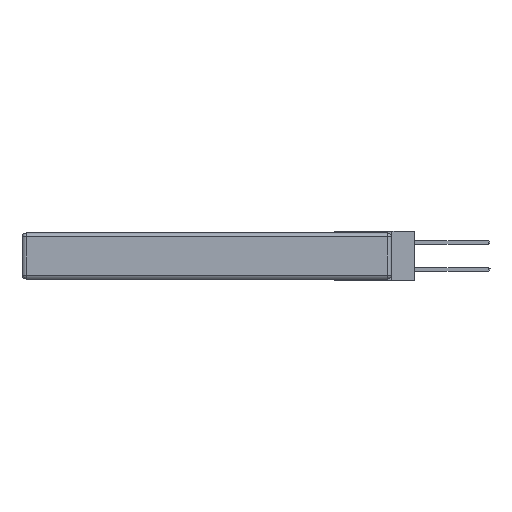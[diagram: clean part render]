
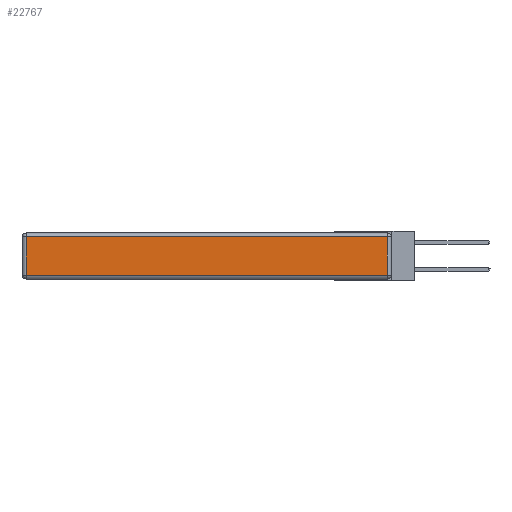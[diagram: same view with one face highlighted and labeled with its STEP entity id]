
A CAD part, left-side view. The second image highlights one B-rep face of the part: STEP entity #22767.
In plain terms, the highlighted planar face has unit normal (-1, 0, 0).
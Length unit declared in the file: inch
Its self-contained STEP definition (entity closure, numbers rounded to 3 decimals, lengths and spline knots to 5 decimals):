
#1443 = VERTEX_POINT ( 'NONE', #26901 ) ;
#3291 = VERTEX_POINT ( 'NONE', #21496 ) ;
#3654 = VECTOR ( 'NONE', #13012, 39.37008 ) ;
#5261 = VERTEX_POINT ( 'NONE', #15467 ) ;
#6190 = EDGE_CURVE ( 'NONE', #3291, #5261, #28071, .T. ) ;
#6710 = PLANE ( 'NONE',  #21973 ) ;
#7044 = CARTESIAN_POINT ( 'NONE',  ( 0., 0., -0.313 ) ) ;
#7120 = DIRECTION ( 'NONE',  ( -1., 0., 0. ) ) ;
#8786 = ORIENTED_EDGE ( 'NONE', *, *, #29482, .T. ) ;
#8874 = EDGE_LOOP ( 'NONE', ( #8786, #17378, #11935, #13070 ) ) ;
#9008 = EDGE_CURVE ( 'NONE', #1443, #3291, #22227, .T. ) ;
#9348 = CARTESIAN_POINT ( 'NONE',  ( 0., 0., -0.343 ) ) ;
#9771 = DIRECTION ( 'NONE',  ( 0., -1., 0. ) ) ;
#11935 = ORIENTED_EDGE ( 'NONE', *, *, #9008, .T. ) ;
#11983 = LINE ( 'NONE', #7044, #22804 ) ;
#13012 = DIRECTION ( 'NONE',  ( 0., 0., 1. ) ) ;
#13070 = ORIENTED_EDGE ( 'NONE', *, *, #6190, .T. ) ;
#13117 = DIRECTION ( 'NONE',  ( 0., 1., 0. ) ) ;
#13322 = CARTESIAN_POINT ( 'NONE',  ( 0., 2.75, -0.03 ) ) ;
#15467 = CARTESIAN_POINT ( 'NONE',  ( 0., 2.72, -0.313 ) ) ;
#17378 = ORIENTED_EDGE ( 'NONE', *, *, #17575, .T. ) ;
#17575 = EDGE_CURVE ( 'NONE', #27498, #1443, #22756, .T. ) ;
#19039 = DIRECTION ( 'NONE',  ( 0., 0., -1. ) ) ;
#21023 = CARTESIAN_POINT ( 'NONE',  ( 0., 2.72, -0.343 ) ) ;
#21474 = VECTOR ( 'NONE', #13117, 39.37008 ) ;
#21496 = CARTESIAN_POINT ( 'NONE',  ( 0., 2.72, -0.03 ) ) ;
#21973 = AXIS2_PLACEMENT_3D ( 'NONE', #9348, #7120, #25855 ) ;
#22227 = LINE ( 'NONE', #13322, #21474 ) ;
#22756 = LINE ( 'NONE', #27522, #3654 ) ;
#22767 = ADVANCED_FACE ( 'NONE', ( #25078 ), #6710, .T. ) ;
#22804 = VECTOR ( 'NONE', #9771, 39.37008 ) ;
#25078 = FACE_OUTER_BOUND ( 'NONE', #8874, .T. ) ;
#25855 = DIRECTION ( 'NONE',  ( 0., 0., 1. ) ) ;
#26560 = VECTOR ( 'NONE', #19039, 39.37008 ) ;
#26901 = CARTESIAN_POINT ( 'NONE',  ( 0., 0.03, -0.03 ) ) ;
#27498 = VERTEX_POINT ( 'NONE', #28935 ) ;
#27522 = CARTESIAN_POINT ( 'NONE',  ( 0., 0.03, -0.343 ) ) ;
#28071 = LINE ( 'NONE', #21023, #26560 ) ;
#28935 = CARTESIAN_POINT ( 'NONE',  ( 0., 0.03, -0.313 ) ) ;
#29482 = EDGE_CURVE ( 'NONE', #5261, #27498, #11983, .T. ) ;
